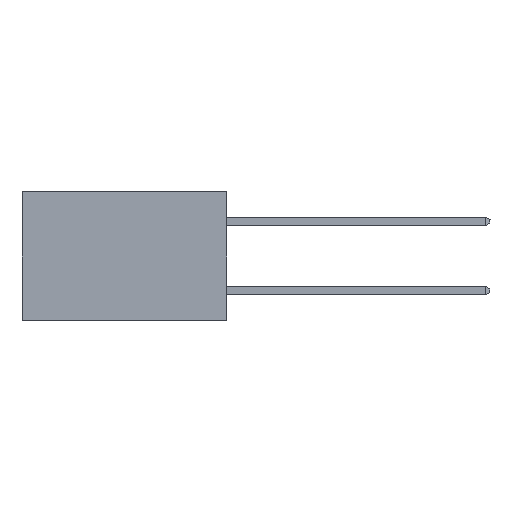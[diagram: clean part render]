
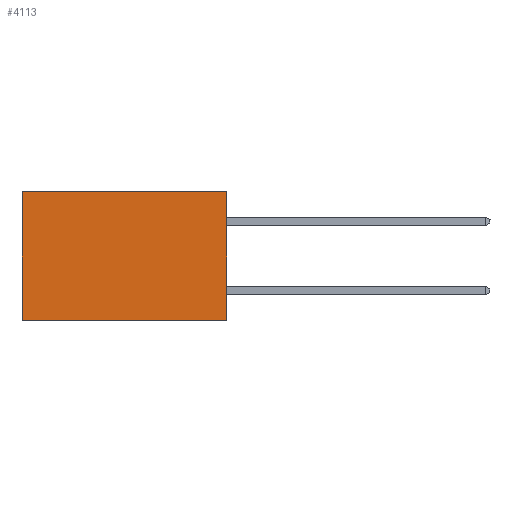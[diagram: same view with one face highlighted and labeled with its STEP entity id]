
A CAD part, left-side view. The second image highlights one B-rep face of the part: STEP entity #4113.
In plain terms, the highlighted planar face has unit normal (-1, 0, 0).
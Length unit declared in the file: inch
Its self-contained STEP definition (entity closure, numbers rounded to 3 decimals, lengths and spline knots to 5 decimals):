
#159 = VERTEX_POINT ( 'NONE', #31916 ) ;
#408 = DIRECTION ( 'NONE',  ( 0., 1., 0. ) ) ;
#760 = CARTESIAN_POINT ( 'NONE',  ( 0.277, 0., 0. ) ) ;
#1787 = CARTESIAN_POINT ( 'NONE',  ( 0.277, 0.59, 0. ) ) ;
#1960 = FACE_OUTER_BOUND ( 'NONE', #30609, .T. ) ;
#2141 = EDGE_CURVE ( 'NONE', #159, #24810, #29182, .T. ) ;
#3277 = DIRECTION ( 'NONE',  ( 0., 1., 0. ) ) ;
#4113 = ADVANCED_FACE ( 'NONE', ( #1960 ), #13303, .F. ) ;
#5073 = VECTOR ( 'NONE', #12350, 39.37008 ) ;
#6457 = EDGE_CURVE ( 'NONE', #13896, #159, #22371, .T. ) ;
#7033 = DIRECTION ( 'NONE',  ( 0., 0., -1. ) ) ;
#7113 = CARTESIAN_POINT ( 'NONE',  ( 0.277, 0., -0.37 ) ) ;
#8016 = VERTEX_POINT ( 'NONE', #1787 ) ;
#8175 = VECTOR ( 'NONE', #7033, 39.37008 ) ;
#8751 = ORIENTED_EDGE ( 'NONE', *, *, #2141, .F. ) ;
#8897 = VECTOR ( 'NONE', #408, 39.37008 ) ;
#9167 = CARTESIAN_POINT ( 'NONE',  ( 0.277, 0.59, -0.37 ) ) ;
#10136 = CARTESIAN_POINT ( 'NONE',  ( 0.277, 0., -0.37 ) ) ;
#11576 = DIRECTION ( 'NONE',  ( 0., 0., -1. ) ) ;
#11612 = DIRECTION ( 'NONE',  ( 1., 0., 0. ) ) ;
#12350 = DIRECTION ( 'NONE',  ( 0., 0., -1. ) ) ;
#12451 = CARTESIAN_POINT ( 'NONE',  ( 0.277, 0., -0.37 ) ) ;
#13303 = PLANE ( 'NONE',  #20568 ) ;
#13896 = VERTEX_POINT ( 'NONE', #760 ) ;
#16129 = ORIENTED_EDGE ( 'NONE', *, *, #24099, .T. ) ;
#17691 = EDGE_CURVE ( 'NONE', #8016, #24810, #20190, .T. ) ;
#19379 = CARTESIAN_POINT ( 'NONE',  ( 0.277, 0., 0. ) ) ;
#20190 = LINE ( 'NONE', #23149, #5073 ) ;
#20568 = AXIS2_PLACEMENT_3D ( 'NONE', #12451, #11612, #11576 ) ;
#22371 = LINE ( 'NONE', #7113, #8175 ) ;
#22665 = ORIENTED_EDGE ( 'NONE', *, *, #6457, .F. ) ;
#23149 = CARTESIAN_POINT ( 'NONE',  ( 0.277, 0.59, -0.37 ) ) ;
#24099 = EDGE_CURVE ( 'NONE', #13896, #8016, #27470, .T. ) ;
#24810 = VERTEX_POINT ( 'NONE', #9167 ) ;
#27470 = LINE ( 'NONE', #19379, #32651 ) ;
#27959 = ORIENTED_EDGE ( 'NONE', *, *, #17691, .T. ) ;
#29182 = LINE ( 'NONE', #10136, #8897 ) ;
#30609 = EDGE_LOOP ( 'NONE', ( #27959, #8751, #22665, #16129 ) ) ;
#31916 = CARTESIAN_POINT ( 'NONE',  ( 0.277, 0., -0.37 ) ) ;
#32651 = VECTOR ( 'NONE', #3277, 39.37008 ) ;
